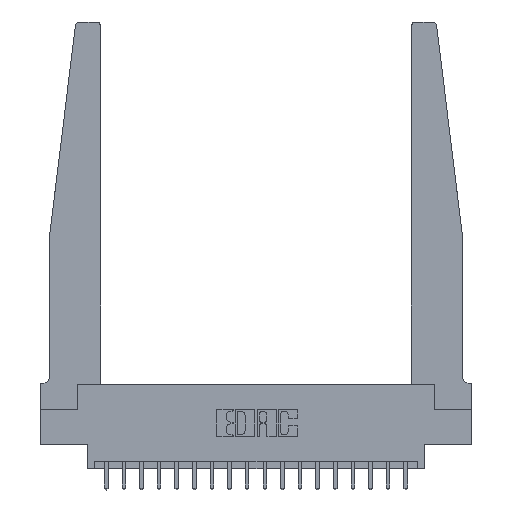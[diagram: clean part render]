
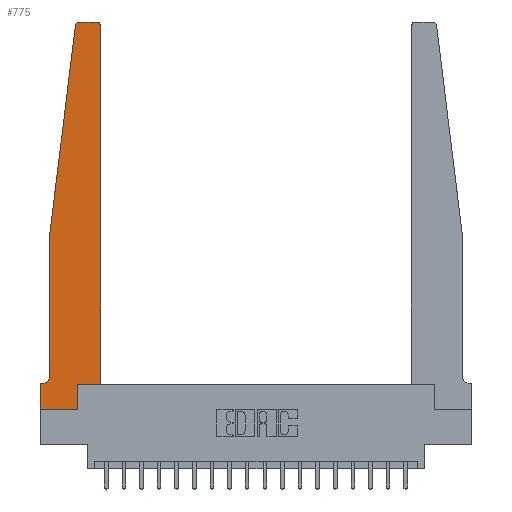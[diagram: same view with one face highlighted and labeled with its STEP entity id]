
A CAD part, top view. The second image highlights one B-rep face of the part: STEP entity #775.
In plain terms, the highlighted planar face has unit normal (0, 0, 1).
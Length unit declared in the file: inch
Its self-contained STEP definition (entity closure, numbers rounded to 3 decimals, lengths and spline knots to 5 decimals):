
#372 = LINE ( 'NONE', #15524, #8273 ) ;
#646 = CARTESIAN_POINT ( 'NONE',  ( 0.425, 0.18, 0.37 ) ) ;
#775 = ADVANCED_FACE ( 'NONE', ( #15805 ), #3819, .T. ) ;
#939 = CIRCLE ( 'NONE', #6386, 0.05 ) ;
#1439 = DIRECTION ( 'NONE',  ( -1., 0., 0. ) ) ;
#1479 = DIRECTION ( 'NONE',  ( 1., 0., 0. ) ) ;
#1521 = VERTEX_POINT ( 'NONE', #13188 ) ;
#1971 = LINE ( 'NONE', #12373, #2497 ) ;
#2401 = LINE ( 'NONE', #2521, #17848 ) ;
#2497 = VECTOR ( 'NONE', #1439, 39.37008 ) ;
#2521 = CARTESIAN_POINT ( 'NONE',  ( 0., 0., 0.37 ) ) ;
#2643 = DIRECTION ( 'NONE',  ( 0., 0., -1. ) ) ;
#2670 = LINE ( 'NONE', #646, #14083 ) ;
#2772 = DIRECTION ( 'NONE',  ( 0., 0., 1. ) ) ;
#3065 = CARTESIAN_POINT ( 'NONE',  ( 0., 0.1875, 0.37 ) ) ;
#3227 = CARTESIAN_POINT ( 'NONE',  ( 0.395, 2.72, 0.37 ) ) ;
#3819 = PLANE ( 'NONE',  #17241 ) ;
#3902 = LINE ( 'NONE', #5289, #19255 ) ;
#4061 = CIRCLE ( 'NONE', #15681, 0.03 ) ;
#4135 = CARTESIAN_POINT ( 'NONE',  ( 0.395, 2.75, 0.37 ) ) ;
#4228 = AXIS2_PLACEMENT_3D ( 'NONE', #5548, #16310, #7156 ) ;
#4281 = CARTESIAN_POINT ( 'NONE',  ( 0.24675, 2.72367, 0.37 ) ) ;
#4330 = EDGE_CURVE ( 'NONE', #11675, #13669, #3902, .T. ) ;
#4787 = DIRECTION ( 'NONE',  ( 1., 0., 0. ) ) ;
#5289 = CARTESIAN_POINT ( 'NONE',  ( 0.2605, 0.18, 0.37 ) ) ;
#5361 = DIRECTION ( 'NONE',  ( 0., 1., 0. ) ) ;
#5548 = CARTESIAN_POINT ( 'NONE',  ( 0.27653, 2.72, 0.37 ) ) ;
#5823 = VERTEX_POINT ( 'NONE', #3065 ) ;
#5938 = VECTOR ( 'NONE', #6603, 39.37008 ) ;
#6109 = CARTESIAN_POINT ( 'NONE',  ( 0.425, 0.18, 0.37 ) ) ;
#6386 = AXIS2_PLACEMENT_3D ( 'NONE', #12012, #2643, #13522 ) ;
#6494 = ORIENTED_EDGE ( 'NONE', *, *, #19133, .T. ) ;
#6603 = DIRECTION ( 'NONE',  ( 0., -1., 0. ) ) ;
#6777 = VERTEX_POINT ( 'NONE', #17940 ) ;
#7156 = DIRECTION ( 'NONE',  ( 1., 0., 0. ) ) ;
#7337 = DIRECTION ( 'NONE',  ( 1., 0., 0. ) ) ;
#7387 = DIRECTION ( 'NONE',  ( -1., 0., 0. ) ) ;
#7917 = DIRECTION ( 'NONE',  ( -0.122, -0.992, 0. ) ) ;
#8200 = CARTESIAN_POINT ( 'NONE',  ( 0., 0., 0.37 ) ) ;
#8264 = ORIENTED_EDGE ( 'NONE', *, *, #15249, .T. ) ;
#8273 = VECTOR ( 'NONE', #7917, 39.37008 ) ;
#8543 = EDGE_CURVE ( 'NONE', #13945, #9674, #939, .T. ) ;
#8937 = VECTOR ( 'NONE', #7387, 39.37008 ) ;
#9253 = ORIENTED_EDGE ( 'NONE', *, *, #4330, .T. ) ;
#9537 = EDGE_CURVE ( 'NONE', #6777, #18587, #2670, .T. ) ;
#9674 = VERTEX_POINT ( 'NONE', #17959 ) ;
#9739 = VERTEX_POINT ( 'NONE', #10535 ) ;
#9947 = CIRCLE ( 'NONE', #4228, 0.03 ) ;
#9972 = EDGE_LOOP ( 'NONE', ( #6494, #13695, #18175, #11077, #17010, #15864, #15570, #8264, #9253, #14156, #15355, #10978 ) ) ;
#10424 = CARTESIAN_POINT ( 'NONE',  ( 0.065, 0.1875, 0.37 ) ) ;
#10535 = CARTESIAN_POINT ( 'NONE',  ( 0.065, 1.25, 0.37 ) ) ;
#10576 = LINE ( 'NONE', #11360, #5938 ) ;
#10738 = DIRECTION ( 'NONE',  ( 0., -1., 0. ) ) ;
#10978 = ORIENTED_EDGE ( 'NONE', *, *, #11264, .T. ) ;
#11021 = LINE ( 'NONE', #6109, #18574 ) ;
#11077 = ORIENTED_EDGE ( 'NONE', *, *, #19359, .T. ) ;
#11238 = EDGE_CURVE ( 'NONE', #15746, #9739, #372, .T. ) ;
#11264 = EDGE_CURVE ( 'NONE', #18587, #12310, #4061, .T. ) ;
#11360 = CARTESIAN_POINT ( 'NONE',  ( 0.065, 1.25, 0.37 ) ) ;
#11664 = CARTESIAN_POINT ( 'NONE',  ( 0.065, 0.2375, 0.37 ) ) ;
#11675 = VERTEX_POINT ( 'NONE', #17953 ) ;
#11727 = CARTESIAN_POINT ( 'NONE',  ( 0., 0.1875, 0.37 ) ) ;
#12012 = CARTESIAN_POINT ( 'NONE',  ( 0.015, 0.2375, 0.37 ) ) ;
#12296 = CARTESIAN_POINT ( 'NONE',  ( 0., 0., 0.37 ) ) ;
#12310 = VERTEX_POINT ( 'NONE', #4135 ) ;
#12373 = CARTESIAN_POINT ( 'NONE',  ( 0.25, 2.75, 0.37 ) ) ;
#12871 = EDGE_CURVE ( 'NONE', #9674, #5823, #17050, .T. ) ;
#13077 = DIRECTION ( 'NONE',  ( 0., 1., 0. ) ) ;
#13188 = CARTESIAN_POINT ( 'NONE',  ( 0.27653, 2.75, 0.37 ) ) ;
#13522 = DIRECTION ( 'NONE',  ( -1., 0., 0. ) ) ;
#13669 = VERTEX_POINT ( 'NONE', #14042 ) ;
#13695 = ORIENTED_EDGE ( 'NONE', *, *, #16860, .T. ) ;
#13945 = VERTEX_POINT ( 'NONE', #11664 ) ;
#14042 = CARTESIAN_POINT ( 'NONE',  ( 0.2605, 0.18, 0.37 ) ) ;
#14068 = DIRECTION ( 'NONE',  ( 0., 0., 1. ) ) ;
#14083 = VECTOR ( 'NONE', #13077, 39.37008 ) ;
#14156 = ORIENTED_EDGE ( 'NONE', *, *, #14874, .T. ) ;
#14419 = VERTEX_POINT ( 'NONE', #8200 ) ;
#14837 = EDGE_CURVE ( 'NONE', #5823, #14419, #19489, .T. ) ;
#14874 = EDGE_CURVE ( 'NONE', #13669, #6777, #11021, .T. ) ;
#15249 = EDGE_CURVE ( 'NONE', #14419, #11675, #2401, .T. ) ;
#15355 = ORIENTED_EDGE ( 'NONE', *, *, #9537, .T. ) ;
#15524 = CARTESIAN_POINT ( 'NONE',  ( 0.065, 1.25, 0.37 ) ) ;
#15528 = VECTOR ( 'NONE', #10738, 39.37008 ) ;
#15570 = ORIENTED_EDGE ( 'NONE', *, *, #14837, .T. ) ;
#15681 = AXIS2_PLACEMENT_3D ( 'NONE', #3227, #14068, #4787 ) ;
#15746 = VERTEX_POINT ( 'NONE', #4281 ) ;
#15805 = FACE_OUTER_BOUND ( 'NONE', #9972, .T. ) ;
#15864 = ORIENTED_EDGE ( 'NONE', *, *, #12871, .T. ) ;
#16310 = DIRECTION ( 'NONE',  ( 0., 0., 1. ) ) ;
#16443 = DIRECTION ( 'NONE',  ( 1., 0., 0. ) ) ;
#16860 = EDGE_CURVE ( 'NONE', #1521, #15746, #9947, .T. ) ;
#17010 = ORIENTED_EDGE ( 'NONE', *, *, #8543, .T. ) ;
#17050 = LINE ( 'NONE', #10424, #8937 ) ;
#17241 = AXIS2_PLACEMENT_3D ( 'NONE', #11727, #2772, #7337 ) ;
#17848 = VECTOR ( 'NONE', #16443, 39.37008 ) ;
#17940 = CARTESIAN_POINT ( 'NONE',  ( 0.425, 0.18, 0.37 ) ) ;
#17953 = CARTESIAN_POINT ( 'NONE',  ( 0.2605, 0., 0.37 ) ) ;
#17959 = CARTESIAN_POINT ( 'NONE',  ( 0.015, 0.1875, 0.37 ) ) ;
#18175 = ORIENTED_EDGE ( 'NONE', *, *, #11238, .T. ) ;
#18574 = VECTOR ( 'NONE', #1479, 39.37008 ) ;
#18587 = VERTEX_POINT ( 'NONE', #18647 ) ;
#18647 = CARTESIAN_POINT ( 'NONE',  ( 0.425, 2.72, 0.37 ) ) ;
#19133 = EDGE_CURVE ( 'NONE', #12310, #1521, #1971, .T. ) ;
#19255 = VECTOR ( 'NONE', #5361, 39.37008 ) ;
#19359 = EDGE_CURVE ( 'NONE', #9739, #13945, #10576, .T. ) ;
#19489 = LINE ( 'NONE', #12296, #15528 ) ;
